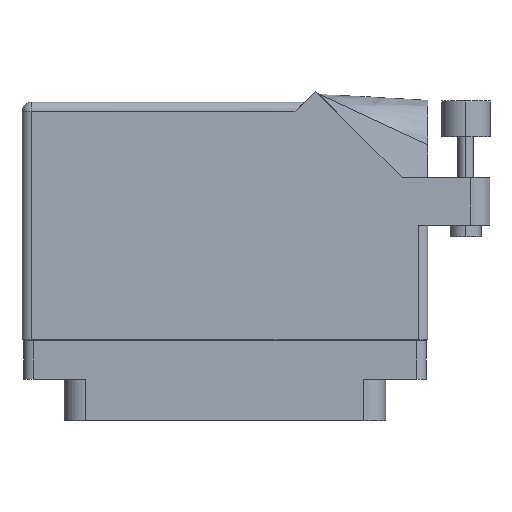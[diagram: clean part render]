
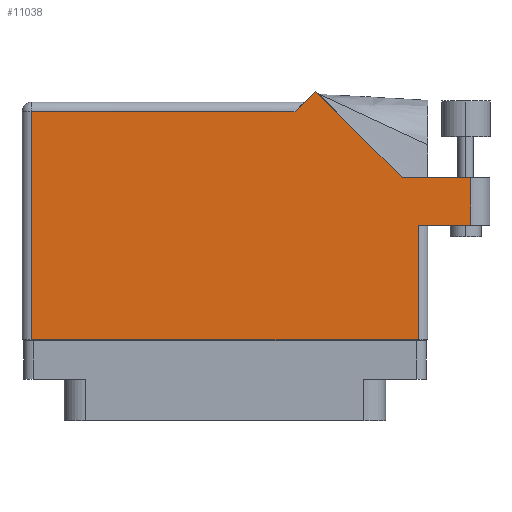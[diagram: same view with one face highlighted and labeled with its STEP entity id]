
A CAD part, front view. The second image highlights one B-rep face of the part: STEP entity #11038.
In plain terms, the highlighted face is planar.
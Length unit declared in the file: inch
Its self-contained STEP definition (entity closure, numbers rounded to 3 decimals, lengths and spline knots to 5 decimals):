
#110 = VERTEX_POINT ( 'NONE', #844 ) ;
#573 = EDGE_CURVE ( 'NONE', #43256, #18834, #2402, .T. ) ;
#765 = CARTESIAN_POINT ( 'NONE',  ( 1.244, 0.637, 0.455 ) ) ;
#844 = CARTESIAN_POINT ( 'NONE',  ( -1.244, -0.1, 0.455 ) ) ;
#1200 = EDGE_CURVE ( 'NONE', #35953, #43256, #34380, .T. ) ;
#1950 = VERTEX_POINT ( 'NONE', #18928 ) ;
#2299 = EDGE_CURVE ( 'NONE', #33745, #35953, #42677, .T. ) ;
#2402 = LINE ( 'NONE', #29991, #31648 ) ;
#4635 = CARTESIAN_POINT ( 'NONE',  ( 0.451, 1.368, 0.455 ) ) ;
#7107 = DIRECTION ( 'NONE',  ( -0.707, 0.707, 0. ) ) ;
#7450 = ORIENTED_EDGE ( 'NONE', *, *, #1200, .T. ) ;
#8586 = CARTESIAN_POINT ( 'NONE',  ( 1.14042, 0.944, 0.455 ) ) ;
#8675 = EDGE_LOOP ( 'NONE', ( #16851, #26078, #7450, #32598, #34331, #15686, #18184, #24377, #38760 ) ) ;
#9039 = LINE ( 'NONE', #765, #36750 ) ;
#9099 = VECTOR ( 'NONE', #34698, 39.37008 ) ;
#11038 = ADVANCED_FACE ( 'NONE', ( #35851 ), #31739, .F. ) ;
#11381 = EDGE_CURVE ( 'NONE', #31553, #110, #35809, .T. ) ;
#12635 = VECTOR ( 'NONE', #30106, 39.37008 ) ;
#13375 = EDGE_CURVE ( 'NONE', #17184, #1950, #9039, .T. ) ;
#14072 = EDGE_CURVE ( 'NONE', #1950, #33745, #43052, .T. ) ;
#15686 = ORIENTED_EDGE ( 'NONE', *, *, #41545, .T. ) ;
#16851 = ORIENTED_EDGE ( 'NONE', *, *, #14072, .T. ) ;
#17022 = CARTESIAN_POINT ( 'NONE',  ( -1.306, 1.368, 0.455 ) ) ;
#17184 = VERTEX_POINT ( 'NONE', #17908 ) ;
#17908 = CARTESIAN_POINT ( 'NONE',  ( 1.244, -0.1, 0.455 ) ) ;
#18184 = ORIENTED_EDGE ( 'NONE', *, *, #11381, .T. ) ;
#18515 = CARTESIAN_POINT ( 'NONE',  ( -1.244, -0.1, 0.455 ) ) ;
#18718 = CARTESIAN_POINT ( 'NONE',  ( -1.306, 1.43, 0.455 ) ) ;
#18834 = VERTEX_POINT ( 'NONE', #32421 ) ;
#18928 = CARTESIAN_POINT ( 'NONE',  ( 1.244, 0.637, 0.455 ) ) ;
#21367 = CARTESIAN_POINT ( 'NONE',  ( 1.581, 0.637, 0.455 ) ) ;
#21386 = CARTESIAN_POINT ( 'NONE',  ( 1.706, 0.944, 0.455 ) ) ;
#21778 = EDGE_CURVE ( 'NONE', #110, #17184, #36808, .T. ) ;
#21818 = VECTOR ( 'NONE', #25000, 39.37008 ) ;
#22081 = DIRECTION ( 'NONE',  ( 0., 1., 0. ) ) ;
#22192 = VECTOR ( 'NONE', #41807, 39.37008 ) ;
#23914 = CARTESIAN_POINT ( 'NONE',  ( -1.306, -0.1, 0.455 ) ) ;
#24377 = ORIENTED_EDGE ( 'NONE', *, *, #21778, .T. ) ;
#25000 = DIRECTION ( 'NONE',  ( -1., 0., 0. ) ) ;
#25261 = DIRECTION ( 'NONE',  ( -1., 0., 0. ) ) ;
#26078 = ORIENTED_EDGE ( 'NONE', *, *, #2299, .T. ) ;
#27122 = DIRECTION ( 'NONE',  ( -1., 0., 0. ) ) ;
#27290 = DIRECTION ( 'NONE',  ( 1., 0., 0. ) ) ;
#27339 = DIRECTION ( 'NONE',  ( 0., 1., 0. ) ) ;
#27900 = VECTOR ( 'NONE', #27290, 39.37008 ) ;
#29991 = CARTESIAN_POINT ( 'NONE',  ( 1.14042, 0.944, 0.455 ) ) ;
#30072 = VECTOR ( 'NONE', #27122, 39.37008 ) ;
#30106 = DIRECTION ( 'NONE',  ( 1., 0., 0. ) ) ;
#30563 = VECTOR ( 'NONE', #22081, 39.37008 ) ;
#31553 = VERTEX_POINT ( 'NONE', #35503 ) ;
#31626 = CARTESIAN_POINT ( 'NONE',  ( 0.513, 1.43, 0.455 ) ) ;
#31627 = LINE ( 'NONE', #17022, #30072 ) ;
#31648 = VECTOR ( 'NONE', #7107, 39.37008 ) ;
#31739 = PLANE ( 'NONE',  #42053 ) ;
#32421 = CARTESIAN_POINT ( 'NONE',  ( 0.58371, 1.50071, 0.455 ) ) ;
#32509 = VERTEX_POINT ( 'NONE', #4635 ) ;
#32598 = ORIENTED_EDGE ( 'NONE', *, *, #573, .T. ) ;
#33745 = VERTEX_POINT ( 'NONE', #21367 ) ;
#34331 = ORIENTED_EDGE ( 'NONE', *, *, #43131, .T. ) ;
#34380 = LINE ( 'NONE', #21386, #21818 ) ;
#34698 = DIRECTION ( 'NONE',  ( -0.707, -0.707, 0. ) ) ;
#34821 = DIRECTION ( 'NONE',  ( 0., 0., -1. ) ) ;
#35503 = CARTESIAN_POINT ( 'NONE',  ( -1.244, 1.368, 0.455 ) ) ;
#35809 = LINE ( 'NONE', #18515, #22192 ) ;
#35851 = FACE_OUTER_BOUND ( 'NONE', #8675, .T. ) ;
#35953 = VERTEX_POINT ( 'NONE', #37269 ) ;
#36274 = LINE ( 'NONE', #31626, #9099 ) ;
#36750 = VECTOR ( 'NONE', #27339, 39.37008 ) ;
#36808 = LINE ( 'NONE', #23914, #27900 ) ;
#37269 = CARTESIAN_POINT ( 'NONE',  ( 1.581, 0.944, 0.455 ) ) ;
#38760 = ORIENTED_EDGE ( 'NONE', *, *, #13375, .T. ) ;
#40826 = CARTESIAN_POINT ( 'NONE',  ( 1.306, 0.637, 0.455 ) ) ;
#41545 = EDGE_CURVE ( 'NONE', #32509, #31553, #31627, .T. ) ;
#41807 = DIRECTION ( 'NONE',  ( 0., -1., 0. ) ) ;
#42053 = AXIS2_PLACEMENT_3D ( 'NONE', #18718, #34821, #25261 ) ;
#42195 = CARTESIAN_POINT ( 'NONE',  ( 1.581, 0.944, 0.455 ) ) ;
#42677 = LINE ( 'NONE', #42195, #30563 ) ;
#43052 = LINE ( 'NONE', #40826, #12635 ) ;
#43131 = EDGE_CURVE ( 'NONE', #18834, #32509, #36274, .T. ) ;
#43256 = VERTEX_POINT ( 'NONE', #8586 ) ;
